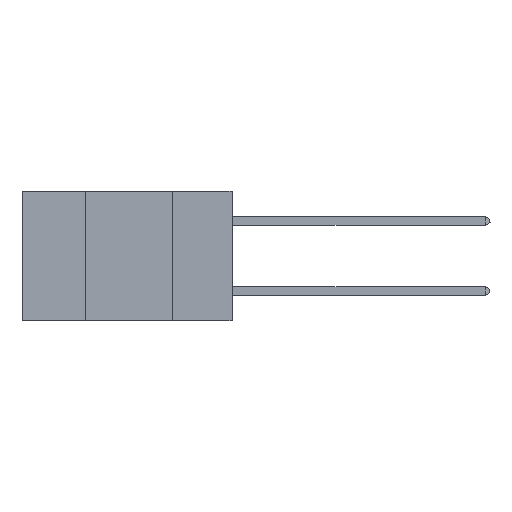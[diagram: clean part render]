
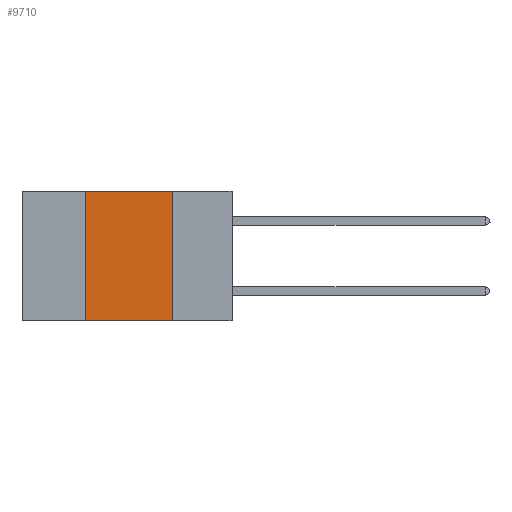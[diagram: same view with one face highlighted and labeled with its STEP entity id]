
A CAD part, left-side view. The second image highlights one B-rep face of the part: STEP entity #9710.
In plain terms, the highlighted planar face has unit normal (-1, 0, 0).
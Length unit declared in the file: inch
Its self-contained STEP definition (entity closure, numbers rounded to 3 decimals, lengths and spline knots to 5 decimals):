
#661 = ORIENTED_EDGE ( 'NONE', *, *, #5586, .F. ) ;
#776 = CARTESIAN_POINT ( 'NONE',  ( 0., 0.6, 0. ) ) ;
#1451 = DIRECTION ( 'NONE',  ( 0., 0., -1. ) ) ;
#1508 = LINE ( 'NONE', #3259, #11205 ) ;
#1519 = LINE ( 'NONE', #776, #10910 ) ;
#1881 = VECTOR ( 'NONE', #2396, 39.37008 ) ;
#1888 = VERTEX_POINT ( 'NONE', #3474 ) ;
#2395 = ORIENTED_EDGE ( 'NONE', *, *, #9798, .F. ) ;
#2396 = DIRECTION ( 'NONE',  ( 0., 0., 1. ) ) ;
#2596 = DIRECTION ( 'NONE',  ( 1., 0., 0. ) ) ;
#3051 = DIRECTION ( 'NONE',  ( 0., -1., 0. ) ) ;
#3259 = CARTESIAN_POINT ( 'NONE',  ( 0., 0.17, 0. ) ) ;
#3325 = CARTESIAN_POINT ( 'NONE',  ( 0., 0.6, 0. ) ) ;
#3474 = CARTESIAN_POINT ( 'NONE',  ( 0., 0.17, 0. ) ) ;
#3611 = CARTESIAN_POINT ( 'NONE',  ( 0., 0.42, -0.37 ) ) ;
#4978 = DIRECTION ( 'NONE',  ( 0., -1., 0. ) ) ;
#5491 = CARTESIAN_POINT ( 'NONE',  ( 0., 0.17, -0.37 ) ) ;
#5541 = VERTEX_POINT ( 'NONE', #5491 ) ;
#5586 = EDGE_CURVE ( 'NONE', #1888, #5541, #1508, .T. ) ;
#5668 = VECTOR ( 'NONE', #3051, 39.37008 ) ;
#5712 = LINE ( 'NONE', #10840, #5668 ) ;
#6914 = PLANE ( 'NONE',  #9827 ) ;
#7480 = VERTEX_POINT ( 'NONE', #3611 ) ;
#7813 = LINE ( 'NONE', #8486, #1881 ) ;
#7969 = CARTESIAN_POINT ( 'NONE',  ( 0., 0.42, 0. ) ) ;
#8099 = EDGE_LOOP ( 'NONE', ( #661, #2395, #9171, #8381 ) ) ;
#8381 = ORIENTED_EDGE ( 'NONE', *, *, #8539, .T. ) ;
#8486 = CARTESIAN_POINT ( 'NONE',  ( 0., 0.42, 0. ) ) ;
#8539 = EDGE_CURVE ( 'NONE', #7480, #5541, #5712, .T. ) ;
#8683 = FACE_OUTER_BOUND ( 'NONE', #8099, .T. ) ;
#9037 = EDGE_CURVE ( 'NONE', #7480, #9622, #7813, .T. ) ;
#9171 = ORIENTED_EDGE ( 'NONE', *, *, #9037, .F. ) ;
#9431 = DIRECTION ( 'NONE',  ( 0., 0., -1. ) ) ;
#9622 = VERTEX_POINT ( 'NONE', #7969 ) ;
#9710 = ADVANCED_FACE ( 'NONE', ( #8683 ), #6914, .F. ) ;
#9798 = EDGE_CURVE ( 'NONE', #9622, #1888, #1519, .T. ) ;
#9827 = AXIS2_PLACEMENT_3D ( 'NONE', #3325, #2596, #9431 ) ;
#10840 = CARTESIAN_POINT ( 'NONE',  ( 0., 0.6, -0.37 ) ) ;
#10910 = VECTOR ( 'NONE', #4978, 39.37008 ) ;
#11205 = VECTOR ( 'NONE', #1451, 39.37008 ) ;
